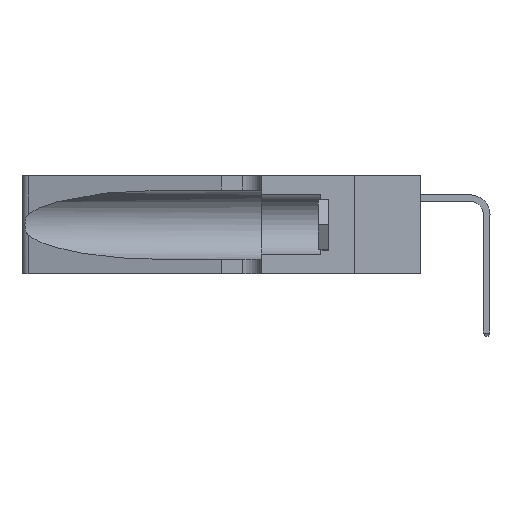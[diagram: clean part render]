
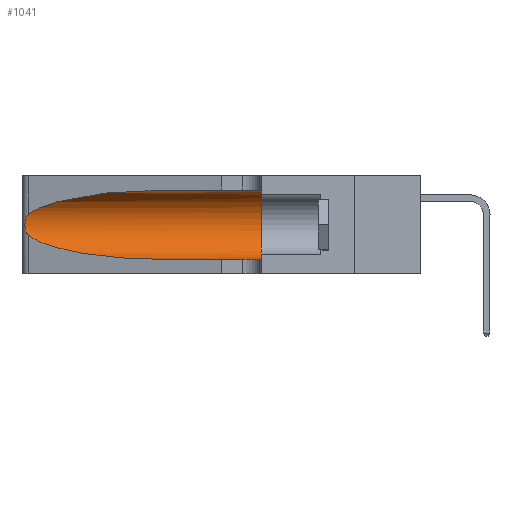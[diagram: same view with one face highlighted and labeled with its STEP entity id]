
A CAD part, left-side view. The second image highlights one B-rep face of the part: STEP entity #1041.
In plain terms, the highlighted cylindrical face has radius 3.308 mm (diameter 6.617 mm), a partial arc.
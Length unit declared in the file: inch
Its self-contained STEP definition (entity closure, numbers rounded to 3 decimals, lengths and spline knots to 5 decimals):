
#337 = DIRECTION ( 'NONE',  ( 0., 0., 1. ) ) ;
#367 =( BOUNDED_CURVE ( )  B_SPLINE_CURVE ( 3, ( #24937, #9620, #31194, #12743 ),
 .UNSPECIFIED., .F., .T. ) 
 B_SPLINE_CURVE_WITH_KNOTS ( ( 4, 4 ),
 ( 3.44316, 4.71239 ),
 .UNSPECIFIED. ) 
 CURVE ( )  GEOMETRIC_REPRESENTATION_ITEM ( )  RATIONAL_B_SPLINE_CURVE ( ( 1., 0.87, 0.87, 1. ) ) 
 REPRESENTATION_ITEM ( '' )  );
#390 = VECTOR ( 'NONE', #10467, 39.37008 ) ;
#562 = CARTESIAN_POINT ( 'NONE',  ( 0.25787, 1.23484, 0.2124 ) ) ;
#1002 = DIRECTION ( 'NONE',  ( 0., 0., -1. ) ) ;
#1041 = ADVANCED_FACE ( 'NONE', ( #34320 ), #33365, .F. ) ;
#2005 = VECTOR ( 'NONE', #9665, 39.37008 ) ;
#3724 = CARTESIAN_POINT ( 'NONE',  ( 0.26018, 1.23835, 0.19895 ) ) ;
#4848 = CARTESIAN_POINT ( 'NONE',  ( 0.1305, 0.35, 0.05475 ) ) ;
#4933 = VERTEX_POINT ( 'NONE', #33721 ) ;
#5575 = ORIENTED_EDGE ( 'NONE', *, *, #23205, .T. ) ;
#5881 = EDGE_CURVE ( 'NONE', #36950, #8571, #24998, .T. ) ;
#6171 = AXIS2_PLACEMENT_3D ( 'NONE', #37351, #18839, #337 ) ;
#6843 = CARTESIAN_POINT ( 'NONE',  ( 0.26075, 1.23896, 0.178 ) ) ;
#7364 = CARTESIAN_POINT ( 'NONE',  ( 0.1305, 1.61858, 0.05475 ) ) ;
#8571 = VERTEX_POINT ( 'NONE', #4848 ) ;
#9532 = CARTESIAN_POINT ( 'NONE',  ( 0.1305, 1.61858, 0.31525 ) ) ;
#9620 = CARTESIAN_POINT ( 'NONE',  ( 0.2373, 1.15595, 0.08982 ) ) ;
#9665 = DIRECTION ( 'NONE',  ( 0., -1., 0. ) ) ;
#9934 = CARTESIAN_POINT ( 'NONE',  ( 0.25856, 1.23593, 0.16098 ) ) ;
#10467 = DIRECTION ( 'NONE',  ( 0., -1., 0. ) ) ;
#10984 = B_SPLINE_CURVE_WITH_KNOTS ( 'NONE', 3,
 ( #34487, #12913, #19068, #562, #22154, #3724, #25240, #6843, #28370, #9934, #31510, #13038, #34612, #16128 ),
 .UNSPECIFIED., .F., .F.,
 ( 4, 2, 2, 2, 2, 2, 4 ),
 ( 0., 0.00027, 0.00053, 0.00107, 0.0016, 0.00187, 0.00214 ),
 .UNSPECIFIED. ) ;
#11455 = VERTEX_POINT ( 'NONE', #39294 ) ;
#11637 = CARTESIAN_POINT ( 'NONE',  ( 0.1305, 0.35, 0.31525 ) ) ;
#12062 = ORIENTED_EDGE ( 'NONE', *, *, #20746, .T. ) ;
#12620 = ORIENTED_EDGE ( 'NONE', *, *, #14414, .T. ) ;
#12704 = VERTEX_POINT ( 'NONE', #16517 ) ;
#12743 = CARTESIAN_POINT ( 'NONE',  ( 0.1305, 0.72297, 0.05475 ) ) ;
#12913 = CARTESIAN_POINT ( 'NONE',  ( 0.25555, 1.22994, 0.2215 ) ) ;
#13038 = CARTESIAN_POINT ( 'NONE',  ( 0.25639, 1.23186, 0.15144 ) ) ;
#13088 = CARTESIAN_POINT ( 'NONE',  ( 0.2373, 1.15595, 0.28018 ) ) ;
#14414 = EDGE_CURVE ( 'NONE', #4933, #11455, #10984, .T. ) ;
#15593 = ORIENTED_EDGE ( 'NONE', *, *, #25898, .F. ) ;
#16050 = CARTESIAN_POINT ( 'NONE',  ( 0.18966, 0.96281, 0.31525 ) ) ;
#16128 = CARTESIAN_POINT ( 'NONE',  ( 0.25487, 1.22718, 0.14631 ) ) ;
#16517 = CARTESIAN_POINT ( 'NONE',  ( 0.1305, 0.72297, 0.31525 ) ) ;
#17529 = EDGE_CURVE ( 'NONE', #12704, #20949, #25629, .T. ) ;
#18839 = DIRECTION ( 'NONE',  ( 0., 1., 0. ) ) ;
#19068 = CARTESIAN_POINT ( 'NONE',  ( 0.25639, 1.23184, 0.21858 ) ) ;
#19470 = DIRECTION ( 'NONE',  ( 0., -1., 0. ) ) ;
#19524 = AXIS2_PLACEMENT_3D ( 'NONE', #22578, #19470, #1002 ) ;
#20746 = EDGE_CURVE ( 'NONE', #11455, #36950, #367, .T. ) ;
#20949 = VERTEX_POINT ( 'NONE', #11637 ) ;
#22154 = CARTESIAN_POINT ( 'NONE',  ( 0.25854, 1.2359, 0.20912 ) ) ;
#22578 = CARTESIAN_POINT ( 'NONE',  ( 0.1305, 1.61858, 0.185 ) ) ;
#23205 = EDGE_CURVE ( 'NONE', #12704, #4933, #25849, .T. ) ;
#24937 = CARTESIAN_POINT ( 'NONE',  ( 0.25487, 1.22718, 0.14631 ) ) ;
#24998 = LINE ( 'NONE', #7364, #390 ) ;
#25240 = CARTESIAN_POINT ( 'NONE',  ( 0.26075, 1.23896, 0.19203 ) ) ;
#25301 = CARTESIAN_POINT ( 'NONE',  ( 0.1305, 0.72297, 0.31525 ) ) ;
#25629 = LINE ( 'NONE', #9532, #2005 ) ;
#25849 =( BOUNDED_CURVE ( )  B_SPLINE_CURVE ( 3, ( #25301, #16050, #13088, #34670 ),
 .UNSPECIFIED., .F., .F. ) 
 B_SPLINE_CURVE_WITH_KNOTS ( ( 4, 4 ),
 ( 1.5708, 2.84003 ),
 .UNSPECIFIED. ) 
 CURVE ( )  GEOMETRIC_REPRESENTATION_ITEM ( )  RATIONAL_B_SPLINE_CURVE ( ( 1., 0.87, 0.87, 1. ) ) 
 REPRESENTATION_ITEM ( '' )  );
#25898 = EDGE_CURVE ( 'NONE', #20949, #8571, #33525, .T. ) ;
#28370 = CARTESIAN_POINT ( 'NONE',  ( 0.26017, 1.23833, 0.17102 ) ) ;
#31194 = CARTESIAN_POINT ( 'NONE',  ( 0.18966, 0.96281, 0.05475 ) ) ;
#31510 = CARTESIAN_POINT ( 'NONE',  ( 0.25789, 1.23486, 0.15765 ) ) ;
#33365 = CYLINDRICAL_SURFACE ( 'NONE', #19524, 0.13025 ) ;
#33525 = CIRCLE ( 'NONE', #6171, 0.13025 ) ;
#33603 = ORIENTED_EDGE ( 'NONE', *, *, #5881, .T. ) ;
#33721 = CARTESIAN_POINT ( 'NONE',  ( 0.25487, 1.22718, 0.22369 ) ) ;
#34320 = FACE_OUTER_BOUND ( 'NONE', #37786, .T. ) ;
#34487 = CARTESIAN_POINT ( 'NONE',  ( 0.25487, 1.22718, 0.22369 ) ) ;
#34612 = CARTESIAN_POINT ( 'NONE',  ( 0.25555, 1.22993, 0.14849 ) ) ;
#34670 = CARTESIAN_POINT ( 'NONE',  ( 0.25487, 1.22718, 0.22369 ) ) ;
#36944 = CARTESIAN_POINT ( 'NONE',  ( 0.1305, 0.72297, 0.05475 ) ) ;
#36950 = VERTEX_POINT ( 'NONE', #36944 ) ;
#37351 = CARTESIAN_POINT ( 'NONE',  ( 0.1305, 0.35, 0.185 ) ) ;
#37786 = EDGE_LOOP ( 'NONE', ( #5575, #12620, #12062, #33603, #15593, #39012 ) ) ;
#39012 = ORIENTED_EDGE ( 'NONE', *, *, #17529, .F. ) ;
#39294 = CARTESIAN_POINT ( 'NONE',  ( 0.25487, 1.22718, 0.14631 ) ) ;
